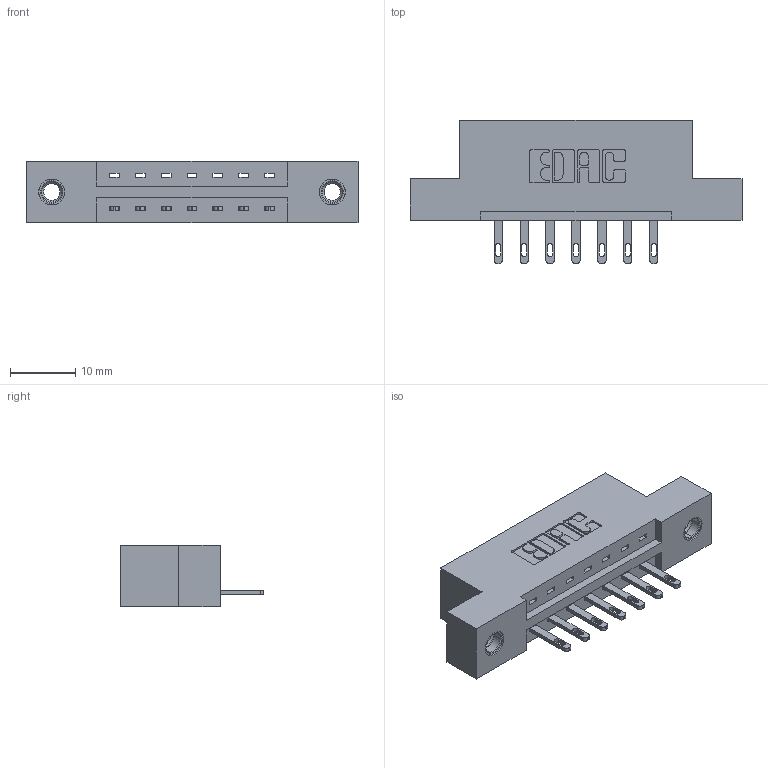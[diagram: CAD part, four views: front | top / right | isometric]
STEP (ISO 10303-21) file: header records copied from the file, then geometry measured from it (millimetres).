
FILE_DESCRIPTION (( 'STEP AP203' ), '1' );
FILE_NAME ('887-007-500-107.STEP', '2020-09-20T15:37:20', ( '' ), ( '' ), 'SwSTEP 2.0', 'SolidWorks 2020', '' );
FILE_SCHEMA (( 'CONFIG_CONTROL_DESIGN' ));
Length unit declared in the file: inch
Products named in the file (4): 887-007-500-107; 345-250-001_345-250-005-103; 345-292-001_345-293-100; 837 Part_Flush Mounting Lugs - 0.156 Dia-TI
Assembly tree (10 placements, depth 2):
  887-007-500-107
    837 Part_Flush Mounting Lugs - 0.156 Dia-TI
    345-292-001_345-293-100  x7
    345-250-001_345-250-005-103  x2
Bounding box: 50.75 x 21.85 x 9.4 mm (x, y, z)
Volume: 4827.4 mm3; surface area: 4851.5 mm2
Topology: 10 solids, 10 shells, 580 faces, 1707 edges, 1130 vertices
Faces by surface type: plane 382, cylinder 182, cone 12, torus 4
Entity records: 10846 total; most frequent: CARTESIAN_POINT 1866, ORIENTED_EDGE 1802, DIRECTION 1677, EDGE_CURVE 901, VECTOR 749, LINE 749, VERTEX_POINT 596, AXIS2_PLACEMENT_3D 464
